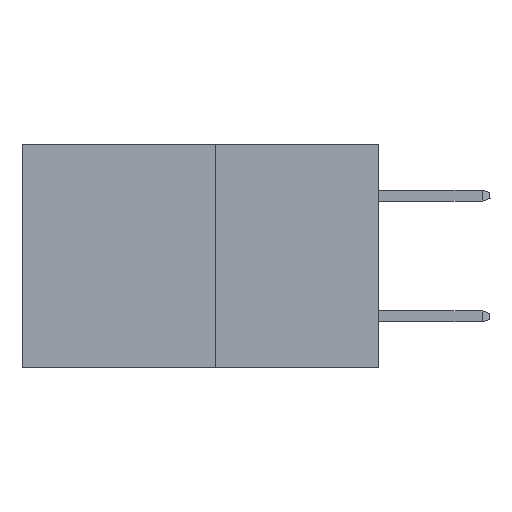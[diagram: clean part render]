
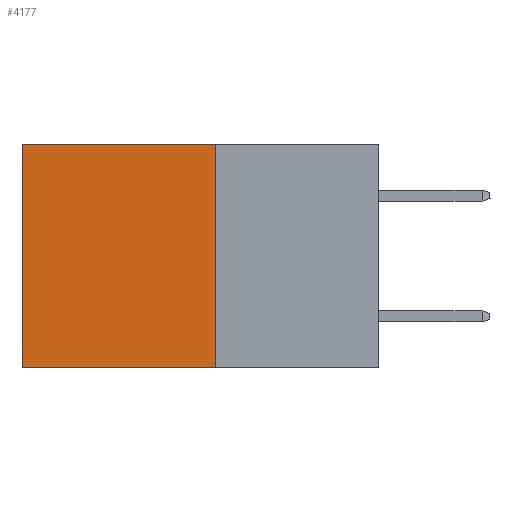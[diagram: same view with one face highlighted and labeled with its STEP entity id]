
A CAD part, left-side view. The second image highlights one B-rep face of the part: STEP entity #4177.
In plain terms, the highlighted planar face has unit normal (-1, 0, 0).
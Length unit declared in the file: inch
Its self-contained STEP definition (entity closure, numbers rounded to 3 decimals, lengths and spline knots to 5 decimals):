
#1972 = DIRECTION ( 'NONE',  ( 0., 0., -1. ) ) ;
#2457 = CARTESIAN_POINT ( 'NONE',  ( 0.277, 0.27, -0.37 ) ) ;
#2647 = VECTOR ( 'NONE', #10456, 39.37008 ) ;
#3343 = LINE ( 'NONE', #16994, #2647 ) ;
#3785 = FACE_OUTER_BOUND ( 'NONE', #27642, .T. ) ;
#4177 = ADVANCED_FACE ( 'NONE', ( #3785 ), #22478, .F. ) ;
#5866 = LINE ( 'NONE', #9771, #18108 ) ;
#5895 = LINE ( 'NONE', #23569, #16773 ) ;
#7179 = DIRECTION ( 'NONE',  ( 1., 0., 0. ) ) ;
#7335 = CARTESIAN_POINT ( 'NONE',  ( 0.277, 0.27, -0.37 ) ) ;
#9771 = CARTESIAN_POINT ( 'NONE',  ( 0.277, 0.27, -0.37 ) ) ;
#10456 = DIRECTION ( 'NONE',  ( 0., 0., -1. ) ) ;
#11148 = VERTEX_POINT ( 'NONE', #24001 ) ;
#12056 = ORIENTED_EDGE ( 'NONE', *, *, #20699, .F. ) ;
#12632 = LINE ( 'NONE', #20840, #17004 ) ;
#13936 = VERTEX_POINT ( 'NONE', #21146 ) ;
#14498 = EDGE_CURVE ( 'NONE', #23594, #11148, #12632, .T. ) ;
#15936 = ORIENTED_EDGE ( 'NONE', *, *, #23845, .T. ) ;
#16773 = VECTOR ( 'NONE', #25743, 39.37008 ) ;
#16909 = ORIENTED_EDGE ( 'NONE', *, *, #14498, .T. ) ;
#16994 = CARTESIAN_POINT ( 'NONE',  ( 0.277, 0.59, -0.37 ) ) ;
#17004 = VECTOR ( 'NONE', #20924, 39.37008 ) ;
#18108 = VECTOR ( 'NONE', #24868, 39.37008 ) ;
#18352 = CARTESIAN_POINT ( 'NONE',  ( 0.277, 0.27, 0. ) ) ;
#20290 = VERTEX_POINT ( 'NONE', #2457 ) ;
#20484 = AXIS2_PLACEMENT_3D ( 'NONE', #7335, #7179, #1972 ) ;
#20699 = EDGE_CURVE ( 'NONE', #23594, #20290, #5895, .T. ) ;
#20840 = CARTESIAN_POINT ( 'NONE',  ( 0.277, 0.27, 0. ) ) ;
#20924 = DIRECTION ( 'NONE',  ( 0., 1., 0. ) ) ;
#21127 = ORIENTED_EDGE ( 'NONE', *, *, #21150, .F. ) ;
#21146 = CARTESIAN_POINT ( 'NONE',  ( 0.277, 0.59, -0.37 ) ) ;
#21150 = EDGE_CURVE ( 'NONE', #20290, #13936, #5866, .T. ) ;
#22478 = PLANE ( 'NONE',  #20484 ) ;
#23569 = CARTESIAN_POINT ( 'NONE',  ( 0.277, 0.27, -0.37 ) ) ;
#23594 = VERTEX_POINT ( 'NONE', #18352 ) ;
#23845 = EDGE_CURVE ( 'NONE', #11148, #13936, #3343, .T. ) ;
#24001 = CARTESIAN_POINT ( 'NONE',  ( 0.277, 0.59, 0. ) ) ;
#24868 = DIRECTION ( 'NONE',  ( 0., 1., 0. ) ) ;
#25743 = DIRECTION ( 'NONE',  ( 0., 0., -1. ) ) ;
#27642 = EDGE_LOOP ( 'NONE', ( #15936, #21127, #12056, #16909 ) ) ;
